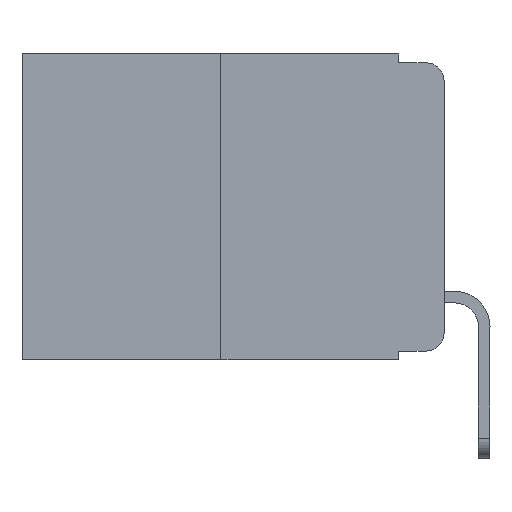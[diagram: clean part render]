
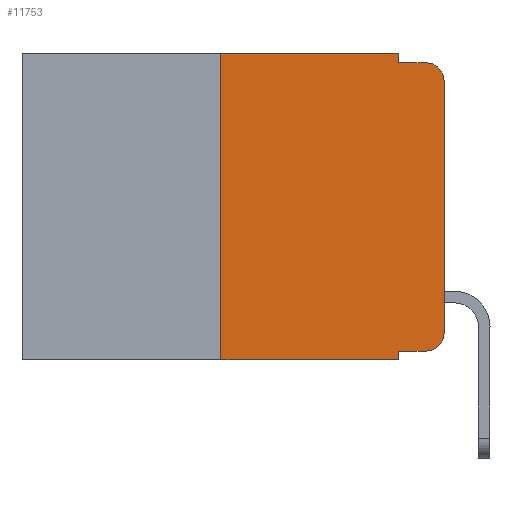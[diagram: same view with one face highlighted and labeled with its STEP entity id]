
A CAD part, left-side view. The second image highlights one B-rep face of the part: STEP entity #11753.
In plain terms, the highlighted planar face has unit normal (-1, 0, 0).
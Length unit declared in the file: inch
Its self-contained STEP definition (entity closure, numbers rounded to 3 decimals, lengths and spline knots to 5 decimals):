
#20 = CARTESIAN_POINT ( 'NONE',  ( 0., 0.25, -0.343 ) ) ;
#250 = CARTESIAN_POINT ( 'NONE',  ( 0., 0., -0.03 ) ) ;
#584 = DIRECTION ( 'NONE',  ( 0., 0., -1. ) ) ;
#990 = CARTESIAN_POINT ( 'NONE',  ( 0., 0.02, -0.01 ) ) ;
#1218 = VERTEX_POINT ( 'NONE', #18667 ) ;
#1300 = VECTOR ( 'NONE', #15221, 39.37008 ) ;
#1605 = FACE_OUTER_BOUND ( 'NONE', #14977, .T. ) ;
#1696 = DIRECTION ( 'NONE',  ( 0., 0., 1. ) ) ;
#1779 = CARTESIAN_POINT ( 'NONE',  ( 0., 0.02, -0.03 ) ) ;
#1807 = ORIENTED_EDGE ( 'NONE', *, *, #13796, .F. ) ;
#1871 = CARTESIAN_POINT ( 'NONE',  ( 0., 0., -0.313 ) ) ;
#1978 = ORIENTED_EDGE ( 'NONE', *, *, #10704, .F. ) ;
#2175 = CARTESIAN_POINT ( 'NONE',  ( 0., 0.473, 0. ) ) ;
#2499 = VERTEX_POINT ( 'NONE', #990 ) ;
#2761 = EDGE_CURVE ( 'NONE', #16170, #14913, #11565, .T. ) ;
#2864 = LINE ( 'NONE', #5954, #17132 ) ;
#3198 = ORIENTED_EDGE ( 'NONE', *, *, #3585, .T. ) ;
#3226 = VECTOR ( 'NONE', #1696, 39.37008 ) ;
#3321 = DIRECTION ( 'NONE',  ( -1., 0., 0. ) ) ;
#3585 = EDGE_CURVE ( 'NONE', #18255, #12130, #11523, .T. ) ;
#3586 = CARTESIAN_POINT ( 'NONE',  ( 0., 0.051, 0. ) ) ;
#5316 = CARTESIAN_POINT ( 'NONE',  ( 0., 0.051, -0.333 ) ) ;
#5436 = VECTOR ( 'NONE', #14580, 39.37008 ) ;
#5559 = DIRECTION ( 'NONE',  ( 0., -1., 0. ) ) ;
#5954 = CARTESIAN_POINT ( 'NONE',  ( 0., 0.051, 0. ) ) ;
#6690 = DIRECTION ( 'NONE',  ( 0., 0., -1. ) ) ;
#6982 = VECTOR ( 'NONE', #584, 39.37008 ) ;
#7145 = CIRCLE ( 'NONE', #11502, 0.02 ) ;
#7544 = CARTESIAN_POINT ( 'NONE',  ( 0., 0.051, -0.343 ) ) ;
#8763 = LINE ( 'NONE', #16134, #11139 ) ;
#8881 = DIRECTION ( 'NONE',  ( 0., 0., -1. ) ) ;
#10397 = ORIENTED_EDGE ( 'NONE', *, *, #15129, .F. ) ;
#10704 = EDGE_CURVE ( 'NONE', #15374, #15078, #8763, .T. ) ;
#10861 = CARTESIAN_POINT ( 'NONE',  ( 0., 0.02, -0.333 ) ) ;
#11059 = LINE ( 'NONE', #3586, #6982 ) ;
#11063 = ORIENTED_EDGE ( 'NONE', *, *, #11931, .T. ) ;
#11120 = ORIENTED_EDGE ( 'NONE', *, *, #17755, .T. ) ;
#11139 = VECTOR ( 'NONE', #5559, 39.37008 ) ;
#11140 = ORIENTED_EDGE ( 'NONE', *, *, #2761, .T. ) ;
#11230 = DIRECTION ( 'NONE',  ( 1., 0., 0. ) ) ;
#11502 = AXIS2_PLACEMENT_3D ( 'NONE', #1779, #3321, #6690 ) ;
#11523 = LINE ( 'NONE', #18792, #16043 ) ;
#11565 = LINE ( 'NONE', #15413, #3226 ) ;
#11753 = ADVANCED_FACE ( 'NONE', ( #1605 ), #14377, .F. ) ;
#11931 = EDGE_CURVE ( 'NONE', #14026, #12980, #13535, .T. ) ;
#12130 = VERTEX_POINT ( 'NONE', #7544 ) ;
#12288 = ORIENTED_EDGE ( 'NONE', *, *, #18117, .F. ) ;
#12507 = CARTESIAN_POINT ( 'NONE',  ( 0., 0.25, 0. ) ) ;
#12980 = VERTEX_POINT ( 'NONE', #10861 ) ;
#13203 = DIRECTION ( 'NONE',  ( 0., 0., -1. ) ) ;
#13261 = ORIENTED_EDGE ( 'NONE', *, *, #18660, .T. ) ;
#13535 = LINE ( 'NONE', #5316, #5436 ) ;
#13766 = CARTESIAN_POINT ( 'NONE',  ( 0., 0.051, -0.01 ) ) ;
#13796 = EDGE_CURVE ( 'NONE', #1218, #2499, #16261, .T. ) ;
#14026 = VERTEX_POINT ( 'NONE', #15732 ) ;
#14062 = CIRCLE ( 'NONE', #19126, 0.02 ) ;
#14183 = CARTESIAN_POINT ( 'NONE',  ( 0., 0.051, 0. ) ) ;
#14377 = PLANE ( 'NONE',  #16332 ) ;
#14504 = EDGE_CURVE ( 'NONE', #18255, #15374, #15831, .T. ) ;
#14580 = DIRECTION ( 'NONE',  ( 0., -1., 0. ) ) ;
#14880 = DIRECTION ( 'NONE',  ( -1., 0., 0. ) ) ;
#14913 = VERTEX_POINT ( 'NONE', #250 ) ;
#14977 = EDGE_LOOP ( 'NONE', ( #11140, #11120, #1807, #10397, #1978, #15007, #3198, #12288, #11063, #13261 ) ) ;
#15007 = ORIENTED_EDGE ( 'NONE', *, *, #14504, .F. ) ;
#15078 = VERTEX_POINT ( 'NONE', #14183 ) ;
#15129 = EDGE_CURVE ( 'NONE', #15078, #1218, #11059, .T. ) ;
#15221 = DIRECTION ( 'NONE',  ( 0., -1., 0. ) ) ;
#15374 = VERTEX_POINT ( 'NONE', #19241 ) ;
#15413 = CARTESIAN_POINT ( 'NONE',  ( 0., 0., 0. ) ) ;
#15732 = CARTESIAN_POINT ( 'NONE',  ( 0., 0.051, -0.333 ) ) ;
#15758 = DIRECTION ( 'NONE',  ( 0., 0., -1. ) ) ;
#15831 = LINE ( 'NONE', #12507, #17939 ) ;
#16043 = VECTOR ( 'NONE', #17217, 39.37008 ) ;
#16134 = CARTESIAN_POINT ( 'NONE',  ( 0., 0.473, 0. ) ) ;
#16170 = VERTEX_POINT ( 'NONE', #1871 ) ;
#16261 = LINE ( 'NONE', #13766, #1300 ) ;
#16332 = AXIS2_PLACEMENT_3D ( 'NONE', #2175, #11230, #15758 ) ;
#17101 = DIRECTION ( 'NONE',  ( 0., 0., 1. ) ) ;
#17132 = VECTOR ( 'NONE', #8881, 39.37008 ) ;
#17217 = DIRECTION ( 'NONE',  ( 0., -1., 0. ) ) ;
#17755 = EDGE_CURVE ( 'NONE', #14913, #2499, #7145, .T. ) ;
#17939 = VECTOR ( 'NONE', #17101, 39.37008 ) ;
#18117 = EDGE_CURVE ( 'NONE', #14026, #12130, #2864, .T. ) ;
#18255 = VERTEX_POINT ( 'NONE', #20 ) ;
#18660 = EDGE_CURVE ( 'NONE', #12980, #16170, #14062, .T. ) ;
#18667 = CARTESIAN_POINT ( 'NONE',  ( 0., 0.051, -0.01 ) ) ;
#18792 = CARTESIAN_POINT ( 'NONE',  ( 0., 0.473, -0.343 ) ) ;
#19126 = AXIS2_PLACEMENT_3D ( 'NONE', #19211, #14880, #13203 ) ;
#19211 = CARTESIAN_POINT ( 'NONE',  ( 0., 0.02, -0.313 ) ) ;
#19241 = CARTESIAN_POINT ( 'NONE',  ( 0., 0.25, 0. ) ) ;
